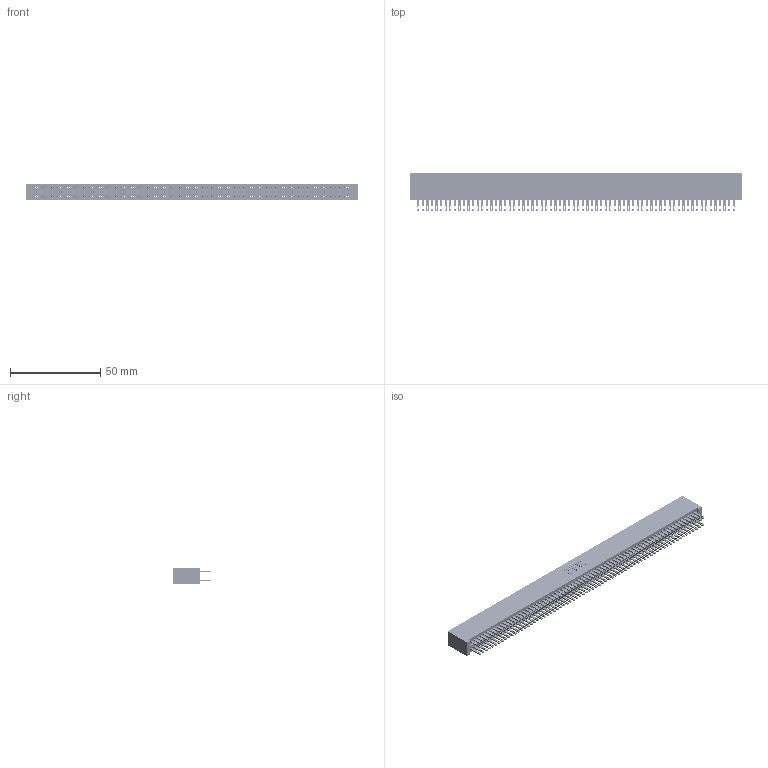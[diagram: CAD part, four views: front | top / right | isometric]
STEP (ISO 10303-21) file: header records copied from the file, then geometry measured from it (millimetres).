
FILE_DESCRIPTION (( 'STEP AP203' ), '1' );
FILE_NAME ('895-140-500-201.STEP', '2020-10-13T19:13:29', ( '' ), ( '' ), 'SwSTEP 2.0', 'SolidWorks 2020', '' );
FILE_SCHEMA (( 'CONFIG_CONTROL_DESIGN' ));
Length unit declared in the file: inch
Products named in the file (3): 845 Part_No Mounting Lugs; 345-292-001_345-293-100; 895-140-500-201
Assembly tree (141 placements, depth 2):
  895-140-500-201
    845 Part_No Mounting Lugs
    345-292-001_345-293-100  x140
Bounding box: 184.4 x 21.51 x 9.4 mm (x, y, z)
Volume: 19216.8 mm3; surface area: 30679.2 mm2
Topology: 141 solids, 141 shells, 6558 faces, 20057 edges, 13370 vertices
Faces by surface type: plane 3856, cylinder 2702
Entity records: 50807 total; most frequent: CARTESIAN_POINT 8488, ORIENTED_EDGE 8422, DIRECTION 7447, EDGE_CURVE 4211, LINE 3803, VECTOR 3803, VERTEX_POINT 2806, AXIS2_PLACEMENT_3D 1822
